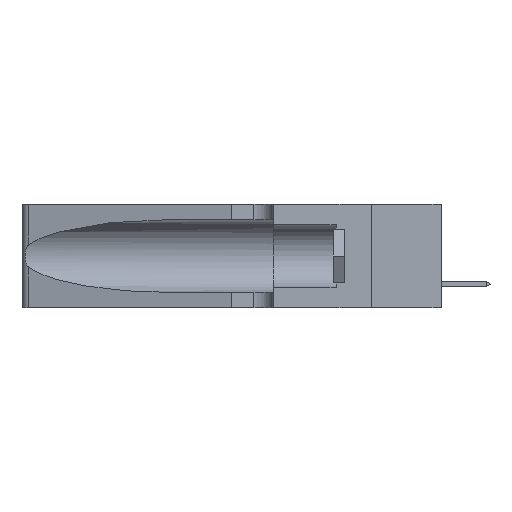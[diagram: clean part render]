
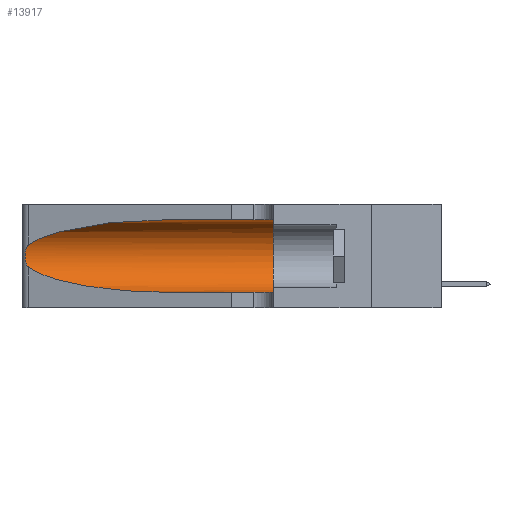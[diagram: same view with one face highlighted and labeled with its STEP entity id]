
A CAD part, left-side view. The second image highlights one B-rep face of the part: STEP entity #13917.
In plain terms, the highlighted cylindrical face has radius 3.308 mm (diameter 6.617 mm), a partial arc.
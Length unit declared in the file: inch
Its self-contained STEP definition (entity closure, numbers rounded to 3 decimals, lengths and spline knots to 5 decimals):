
#44 = EDGE_CURVE ( 'NONE', #13964, #1317, #18909, .T. ) ;
#119 = CARTESIAN_POINT ( 'NONE',  ( 0.18966, 0.96281, 0.31525 ) ) ;
#203 = CARTESIAN_POINT ( 'NONE',  ( 0.25487, 1.22718, 0.22369 ) ) ;
#478 = CARTESIAN_POINT ( 'NONE',  ( 0.25856, 1.23593, 0.16098 ) ) ;
#695 = CARTESIAN_POINT ( 'NONE',  ( 0.26018, 1.23835, 0.19895 ) ) ;
#701 = VECTOR ( 'NONE', #10397, 39.37008 ) ;
#1317 = VERTEX_POINT ( 'NONE', #11502 ) ;
#1944 =( BOUNDED_CURVE ( )  B_SPLINE_CURVE ( 3, ( #5062, #119, #11247, #203 ),
 .UNSPECIFIED., .F., .T. ) 
 B_SPLINE_CURVE_WITH_KNOTS ( ( 4, 4 ),
 ( 1.5708, 2.84003 ),
 .UNSPECIFIED. ) 
 CURVE ( )  GEOMETRIC_REPRESENTATION_ITEM ( )  RATIONAL_B_SPLINE_CURVE ( ( 1., 0.87, 0.87, 1. ) ) 
 REPRESENTATION_ITEM ( '' )  );
#2334 = CARTESIAN_POINT ( 'NONE',  ( 0.25639, 1.23186, 0.15144 ) ) ;
#2801 = DIRECTION ( 'NONE',  ( 0., 0., -1. ) ) ;
#3978 = CARTESIAN_POINT ( 'NONE',  ( 0.25487, 1.22718, 0.14631 ) ) ;
#4167 =( BOUNDED_CURVE ( )  B_SPLINE_CURVE ( 3, ( #6188, #10966, #6584, #6459 ),
 .UNSPECIFIED., .F., .T. ) 
 B_SPLINE_CURVE_WITH_KNOTS ( ( 4, 4 ),
 ( 3.44316, 4.71239 ),
 .UNSPECIFIED. ) 
 CURVE ( )  GEOMETRIC_REPRESENTATION_ITEM ( )  RATIONAL_B_SPLINE_CURVE ( ( 1., 0.87, 0.87, 1. ) ) 
 REPRESENTATION_ITEM ( '' )  );
#4574 = DIRECTION ( 'NONE',  ( 0., 1., 0. ) ) ;
#4586 = CARTESIAN_POINT ( 'NONE',  ( 0.1305, 1.61858, 0.185 ) ) ;
#5062 = CARTESIAN_POINT ( 'NONE',  ( 0.1305, 0.72297, 0.31525 ) ) ;
#5239 = ORIENTED_EDGE ( 'NONE', *, *, #11899, .T. ) ;
#5242 = CARTESIAN_POINT ( 'NONE',  ( 0.1305, 0.35, 0.05475 ) ) ;
#5474 = CARTESIAN_POINT ( 'NONE',  ( 0.25787, 1.23484, 0.2124 ) ) ;
#5556 = LINE ( 'NONE', #8015, #9339 ) ;
#5909 = EDGE_CURVE ( 'NONE', #17928, #12472, #11009, .T. ) ;
#5958 = AXIS2_PLACEMENT_3D ( 'NONE', #4586, #6205, #2801 ) ;
#5982 = DIRECTION ( 'NONE',  ( 0., 0., 1. ) ) ;
#6188 = CARTESIAN_POINT ( 'NONE',  ( 0.25487, 1.22718, 0.14631 ) ) ;
#6205 = DIRECTION ( 'NONE',  ( 0., -1., 0. ) ) ;
#6459 = CARTESIAN_POINT ( 'NONE',  ( 0.1305, 0.72297, 0.05475 ) ) ;
#6584 = CARTESIAN_POINT ( 'NONE',  ( 0.18966, 0.96281, 0.05475 ) ) ;
#6937 = VERTEX_POINT ( 'NONE', #15601 ) ;
#7006 = CARTESIAN_POINT ( 'NONE',  ( 0.26075, 1.23896, 0.19203 ) ) ;
#7069 = CARTESIAN_POINT ( 'NONE',  ( 0.25555, 1.22993, 0.14849 ) ) ;
#7138 = CARTESIAN_POINT ( 'NONE',  ( 0.25555, 1.22994, 0.2215 ) ) ;
#7256 = AXIS2_PLACEMENT_3D ( 'NONE', #7788, #4574, #5982 ) ;
#7750 = FACE_OUTER_BOUND ( 'NONE', #15027, .T. ) ;
#7788 = CARTESIAN_POINT ( 'NONE',  ( 0.1305, 0.35, 0.185 ) ) ;
#7946 = DIRECTION ( 'NONE',  ( 0., -1., 0. ) ) ;
#8015 = CARTESIAN_POINT ( 'NONE',  ( 0.1305, 1.61858, 0.05475 ) ) ;
#8841 = CARTESIAN_POINT ( 'NONE',  ( 0.26017, 1.23833, 0.17102 ) ) ;
#9339 = VECTOR ( 'NONE', #7946, 39.37008 ) ;
#9535 = CYLINDRICAL_SURFACE ( 'NONE', #5958, 0.13025 ) ;
#10396 = CARTESIAN_POINT ( 'NONE',  ( 0.25639, 1.23184, 0.21858 ) ) ;
#10397 = DIRECTION ( 'NONE',  ( 0., -1., 0. ) ) ;
#10587 = CIRCLE ( 'NONE', #7256, 0.13025 ) ;
#10623 = EDGE_CURVE ( 'NONE', #12472, #6937, #4167, .T. ) ;
#10627 = EDGE_CURVE ( 'NONE', #13964, #17928, #1944, .T. ) ;
#10909 = CARTESIAN_POINT ( 'NONE',  ( 0.1305, 0.72297, 0.31525 ) ) ;
#10966 = CARTESIAN_POINT ( 'NONE',  ( 0.2373, 1.15595, 0.08982 ) ) ;
#10968 = ORIENTED_EDGE ( 'NONE', *, *, #10623, .T. ) ;
#11009 = B_SPLINE_CURVE_WITH_KNOTS ( 'NONE', 3,
 ( #15048, #7138, #10396, #5474, #13433, #695, #7006, #13515, #8841, #478, #13370, #2334, #7069, #3978 ),
 .UNSPECIFIED., .F., .F.,
 ( 4, 2, 2, 2, 2, 2, 4 ),
 ( 0., 0.00027, 0.00053, 0.00107, 0.0016, 0.00187, 0.00214 ),
 .UNSPECIFIED. ) ;
#11247 = CARTESIAN_POINT ( 'NONE',  ( 0.2373, 1.15595, 0.28018 ) ) ;
#11502 = CARTESIAN_POINT ( 'NONE',  ( 0.1305, 0.35, 0.31525 ) ) ;
#11899 = EDGE_CURVE ( 'NONE', #6937, #13070, #5556, .T. ) ;
#11941 = CARTESIAN_POINT ( 'NONE',  ( 0.1305, 1.61858, 0.31525 ) ) ;
#12256 = EDGE_CURVE ( 'NONE', #1317, #13070, #10587, .T. ) ;
#12472 = VERTEX_POINT ( 'NONE', #16124 ) ;
#13070 = VERTEX_POINT ( 'NONE', #5242 ) ;
#13370 = CARTESIAN_POINT ( 'NONE',  ( 0.25789, 1.23486, 0.15765 ) ) ;
#13433 = CARTESIAN_POINT ( 'NONE',  ( 0.25854, 1.2359, 0.20912 ) ) ;
#13515 = CARTESIAN_POINT ( 'NONE',  ( 0.26075, 1.23896, 0.178 ) ) ;
#13917 = ADVANCED_FACE ( 'NONE', ( #7750 ), #9535, .F. ) ;
#13964 = VERTEX_POINT ( 'NONE', #10909 ) ;
#15027 = EDGE_LOOP ( 'NONE', ( #19036, #18282, #10968, #5239, #15284, #16718 ) ) ;
#15048 = CARTESIAN_POINT ( 'NONE',  ( 0.25487, 1.22718, 0.22369 ) ) ;
#15284 = ORIENTED_EDGE ( 'NONE', *, *, #12256, .F. ) ;
#15601 = CARTESIAN_POINT ( 'NONE',  ( 0.1305, 0.72297, 0.05475 ) ) ;
#16124 = CARTESIAN_POINT ( 'NONE',  ( 0.25487, 1.22718, 0.14631 ) ) ;
#16718 = ORIENTED_EDGE ( 'NONE', *, *, #44, .F. ) ;
#17116 = CARTESIAN_POINT ( 'NONE',  ( 0.25487, 1.22718, 0.22369 ) ) ;
#17928 = VERTEX_POINT ( 'NONE', #17116 ) ;
#18282 = ORIENTED_EDGE ( 'NONE', *, *, #5909, .T. ) ;
#18909 = LINE ( 'NONE', #11941, #701 ) ;
#19036 = ORIENTED_EDGE ( 'NONE', *, *, #10627, .T. ) ;
